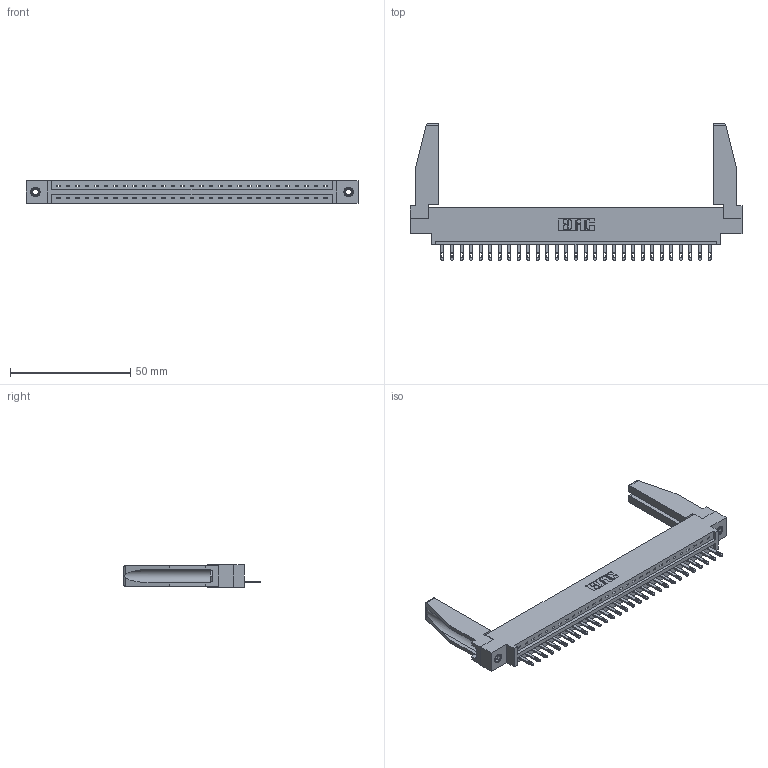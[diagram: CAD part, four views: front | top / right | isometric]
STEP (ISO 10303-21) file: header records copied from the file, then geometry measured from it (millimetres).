
FILE_DESCRIPTION (( 'STEP AP203' ), '1' );
FILE_NAME ('337-029-500-678.STEP', '2019-09-30T21:46:49', ( '' ), ( '' ), 'SwSTEP 2.0', 'SolidWorks 2016', '' );
FILE_SCHEMA (( 'CONFIG_CONTROL_DESIGN' ));
Length unit declared in the file: inch
Products named in the file (5): 345-292-001_345-293-100; 337-029-500-678; 307-220-078; 337 Part_0.170 Offset - 0.156 Dia-TI; 345-250-001_345-250-001-102
Assembly tree (34 placements, depth 2):
  337-029-500-678
    337 Part_0.170 Offset - 0.156 Dia-TI
    345-292-001_345-293-100  x29
    345-250-001_345-250-001-102  x2
    307-220-078  x2
Bounding box: 137.92 x 56.65 x 9.4 mm (x, y, z)
Volume: 18065.8 mm3; surface area: 18470.7 mm2
Topology: 34 solids, 34 shells, 1930 faces, 5873 edges, 3906 vertices
Faces by surface type: plane 1318, cylinder 596, cone 12, torus 4
Entity records: 25740 total; most frequent: CARTESIAN_POINT 4475, ORIENTED_EDGE 4396, DIRECTION 3804, EDGE_CURVE 2198, VECTOR 2028, LINE 2028, VERTEX_POINT 1460, AXIS2_PLACEMENT_3D 888
